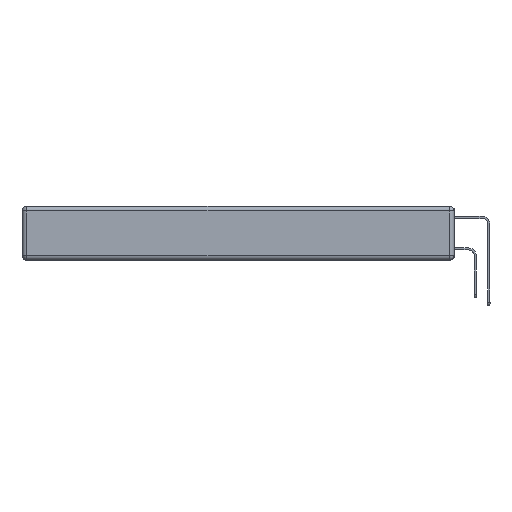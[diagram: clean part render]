
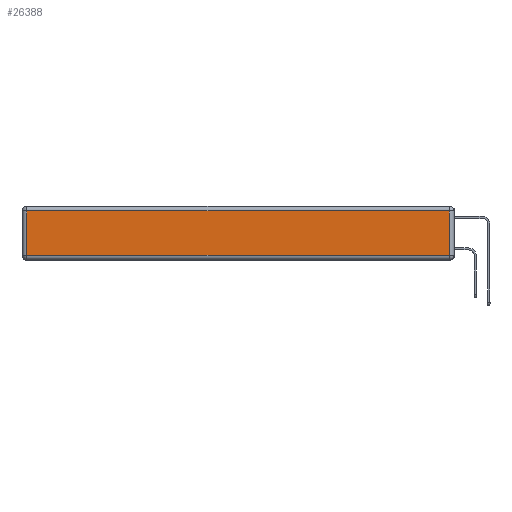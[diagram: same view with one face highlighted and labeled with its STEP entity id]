
A CAD part, left-side view. The second image highlights one B-rep face of the part: STEP entity #26388.
In plain terms, the highlighted planar face has unit normal (-1, 0, 0).
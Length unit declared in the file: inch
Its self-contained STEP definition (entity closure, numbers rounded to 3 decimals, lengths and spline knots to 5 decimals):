
#1089 = CARTESIAN_POINT ( 'NONE',  ( 0., 2.72, -0.313 ) ) ;
#1617 = LINE ( 'NONE', #24721, #25426 ) ;
#2096 = VERTEX_POINT ( 'NONE', #8049 ) ;
#2144 = LINE ( 'NONE', #16808, #22724 ) ;
#2744 = CARTESIAN_POINT ( 'NONE',  ( 0., 2.75, -0.03 ) ) ;
#3752 = DIRECTION ( 'NONE',  ( 0., 0., 1. ) ) ;
#5583 = VERTEX_POINT ( 'NONE', #13428 ) ;
#5948 = EDGE_LOOP ( 'NONE', ( #9069, #8144, #9344, #6499 ) ) ;
#6309 = DIRECTION ( 'NONE',  ( 0., 1., 0. ) ) ;
#6499 = ORIENTED_EDGE ( 'NONE', *, *, #14350, .T. ) ;
#7920 = VECTOR ( 'NONE', #20792, 39.37008 ) ;
#8049 = CARTESIAN_POINT ( 'NONE',  ( 0., 2.72, -0.03 ) ) ;
#8144 = ORIENTED_EDGE ( 'NONE', *, *, #8567, .T. ) ;
#8181 = DIRECTION ( 'NONE',  ( 0., 0., 1. ) ) ;
#8226 = LINE ( 'NONE', #16574, #7920 ) ;
#8567 = EDGE_CURVE ( 'NONE', #5583, #13777, #1617, .T. ) ;
#9069 = ORIENTED_EDGE ( 'NONE', *, *, #9848, .T. ) ;
#9344 = ORIENTED_EDGE ( 'NONE', *, *, #23238, .T. ) ;
#9770 = PLANE ( 'NONE',  #23285 ) ;
#9848 = EDGE_CURVE ( 'NONE', #14427, #5583, #2144, .T. ) ;
#13428 = CARTESIAN_POINT ( 'NONE',  ( 0., 0.03, -0.313 ) ) ;
#13777 = VERTEX_POINT ( 'NONE', #20952 ) ;
#14146 = FACE_OUTER_BOUND ( 'NONE', #5948, .T. ) ;
#14350 = EDGE_CURVE ( 'NONE', #2096, #14427, #8226, .T. ) ;
#14427 = VERTEX_POINT ( 'NONE', #1089 ) ;
#16574 = CARTESIAN_POINT ( 'NONE',  ( 0., 2.72, -0.343 ) ) ;
#16808 = CARTESIAN_POINT ( 'NONE',  ( 0., 0., -0.313 ) ) ;
#18133 = CARTESIAN_POINT ( 'NONE',  ( 0., 0., -0.343 ) ) ;
#20792 = DIRECTION ( 'NONE',  ( 0., 0., -1. ) ) ;
#20952 = CARTESIAN_POINT ( 'NONE',  ( 0., 0.03, -0.03 ) ) ;
#21469 = LINE ( 'NONE', #2744, #22280 ) ;
#22280 = VECTOR ( 'NONE', #6309, 39.37008 ) ;
#22724 = VECTOR ( 'NONE', #23344, 39.37008 ) ;
#23238 = EDGE_CURVE ( 'NONE', #13777, #2096, #21469, .T. ) ;
#23285 = AXIS2_PLACEMENT_3D ( 'NONE', #18133, #26431, #3752 ) ;
#23344 = DIRECTION ( 'NONE',  ( 0., -1., 0. ) ) ;
#24721 = CARTESIAN_POINT ( 'NONE',  ( 0., 0.03, -0.343 ) ) ;
#25426 = VECTOR ( 'NONE', #8181, 39.37008 ) ;
#26388 = ADVANCED_FACE ( 'NONE', ( #14146 ), #9770, .T. ) ;
#26431 = DIRECTION ( 'NONE',  ( -1., 0., 0. ) ) ;
